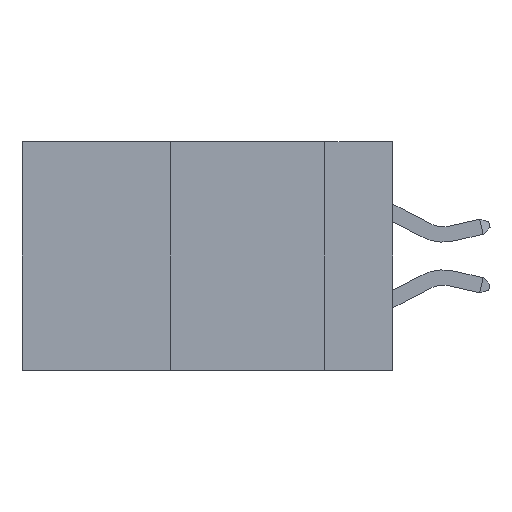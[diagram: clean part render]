
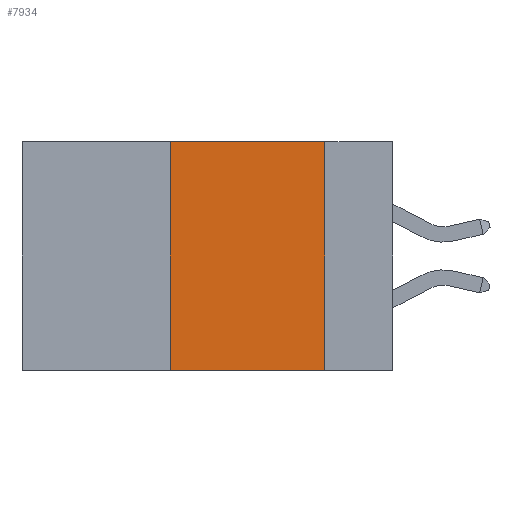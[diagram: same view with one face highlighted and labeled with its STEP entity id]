
A CAD part, left-side view. The second image highlights one B-rep face of the part: STEP entity #7934.
In plain terms, the highlighted planar face has unit normal (-1, 0, 0).
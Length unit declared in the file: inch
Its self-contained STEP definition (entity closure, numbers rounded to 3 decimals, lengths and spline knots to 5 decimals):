
#43 = VERTEX_POINT ( 'NONE', #5727 ) ;
#97 = EDGE_CURVE ( 'NONE', #4627, #4753, #285, .T. ) ;
#176 = EDGE_CURVE ( 'NONE', #43, #4627, #1461, .T. ) ;
#285 = LINE ( 'NONE', #4290, #12454 ) ;
#1368 = VECTOR ( 'NONE', #3242, 39.37008 ) ;
#1461 = LINE ( 'NONE', #11472, #1368 ) ;
#1574 = ORIENTED_EDGE ( 'NONE', *, *, #12754, .T. ) ;
#1575 = VECTOR ( 'NONE', #2024, 39.37008 ) ;
#1992 = VECTOR ( 'NONE', #6702, 39.37008 ) ;
#2024 = DIRECTION ( 'NONE',  ( 0., 0., -1. ) ) ;
#2669 = ORIENTED_EDGE ( 'NONE', *, *, #97, .F. ) ;
#2759 = VERTEX_POINT ( 'NONE', #8204 ) ;
#3096 = FACE_OUTER_BOUND ( 'NONE', #8140, .T. ) ;
#3160 = DIRECTION ( 'NONE',  ( 0., 0., -1. ) ) ;
#3242 = DIRECTION ( 'NONE',  ( 0., 0., 1. ) ) ;
#4280 = DIRECTION ( 'NONE',  ( 1., 0., 0. ) ) ;
#4290 = CARTESIAN_POINT ( 'NONE',  ( 0., 0.6, 0. ) ) ;
#4627 = VERTEX_POINT ( 'NONE', #9186 ) ;
#4753 = VERTEX_POINT ( 'NONE', #11166 ) ;
#5727 = CARTESIAN_POINT ( 'NONE',  ( 0., 0.36, -0.37 ) ) ;
#6501 = AXIS2_PLACEMENT_3D ( 'NONE', #7970, #4280, #3160 ) ;
#6702 = DIRECTION ( 'NONE',  ( 0., -1., 0. ) ) ;
#7934 = ADVANCED_FACE ( 'NONE', ( #3096 ), #11263, .F. ) ;
#7970 = CARTESIAN_POINT ( 'NONE',  ( 0., 0.6, 0. ) ) ;
#8140 = EDGE_LOOP ( 'NONE', ( #8951, #2669, #9289, #1574 ) ) ;
#8200 = EDGE_CURVE ( 'NONE', #4753, #2759, #10121, .T. ) ;
#8204 = CARTESIAN_POINT ( 'NONE',  ( 0., 0.11, -0.37 ) ) ;
#8951 = ORIENTED_EDGE ( 'NONE', *, *, #8200, .F. ) ;
#9186 = CARTESIAN_POINT ( 'NONE',  ( 0., 0.36, 0. ) ) ;
#9289 = ORIENTED_EDGE ( 'NONE', *, *, #176, .F. ) ;
#10121 = LINE ( 'NONE', #11043, #1575 ) ;
#10877 = CARTESIAN_POINT ( 'NONE',  ( 0., 0.6, -0.37 ) ) ;
#11043 = CARTESIAN_POINT ( 'NONE',  ( 0., 0.11, 0. ) ) ;
#11166 = CARTESIAN_POINT ( 'NONE',  ( 0., 0.11, 0. ) ) ;
#11263 = PLANE ( 'NONE',  #6501 ) ;
#11269 = DIRECTION ( 'NONE',  ( 0., -1., 0. ) ) ;
#11472 = CARTESIAN_POINT ( 'NONE',  ( 0., 0.36, 0. ) ) ;
#11751 = LINE ( 'NONE', #10877, #1992 ) ;
#12454 = VECTOR ( 'NONE', #11269, 39.37008 ) ;
#12754 = EDGE_CURVE ( 'NONE', #43, #2759, #11751, .T. ) ;
